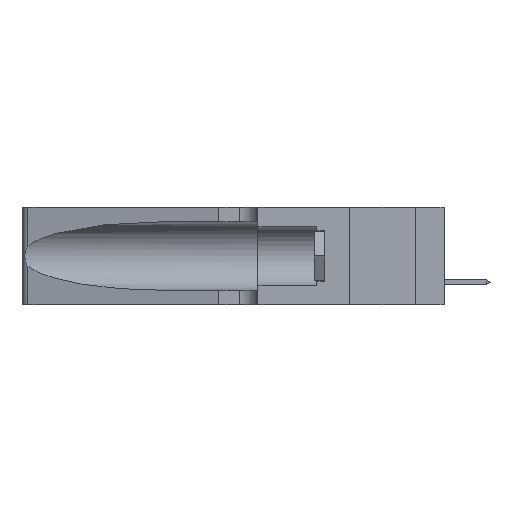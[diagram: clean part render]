
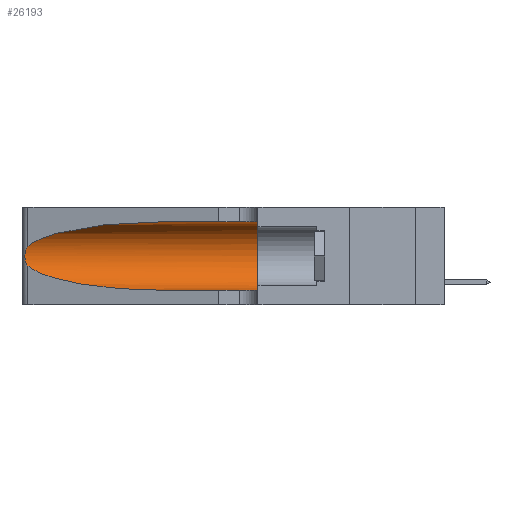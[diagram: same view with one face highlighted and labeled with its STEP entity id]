
A CAD part, left-side view. The second image highlights one B-rep face of the part: STEP entity #26193.
In plain terms, the highlighted cylindrical face has radius 3.308 mm (diameter 6.617 mm), a partial arc.
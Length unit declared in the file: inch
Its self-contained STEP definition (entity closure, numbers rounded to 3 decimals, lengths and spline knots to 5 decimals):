
#1196 = DIRECTION ( 'NONE',  ( 0., 0., -1. ) ) ;
#1380 = VERTEX_POINT ( 'NONE', #15927 ) ;
#1397 = CARTESIAN_POINT ( 'NONE',  ( 0.1305, 1.61858, 0.185 ) ) ;
#1692 = CARTESIAN_POINT ( 'NONE',  ( 0.26075, 1.23896, 0.19203 ) ) ;
#4645 = DIRECTION ( 'NONE',  ( 0., 0., 1. ) ) ;
#4853 = CYLINDRICAL_SURFACE ( 'NONE', #7527, 0.13025 ) ;
#5171 = CIRCLE ( 'NONE', #34325, 0.13025 ) ;
#5528 = DIRECTION ( 'NONE',  ( 0., -1., 0. ) ) ;
#6163 = FACE_OUTER_BOUND ( 'NONE', #28366, .T. ) ;
#6665 = CARTESIAN_POINT ( 'NONE',  ( 0.25487, 1.22718, 0.14631 ) ) ;
#7006 = ORIENTED_EDGE ( 'NONE', *, *, #47907, .F. ) ;
#7014 = CARTESIAN_POINT ( 'NONE',  ( 0.1305, 0.72297, 0.05475 ) ) ;
#7527 = AXIS2_PLACEMENT_3D ( 'NONE', #1397, #5528, #1196 ) ;
#8422 = VECTOR ( 'NONE', #16649, 39.37008 ) ;
#8935 = ORIENTED_EDGE ( 'NONE', *, *, #40357, .T. ) ;
#9298 = CARTESIAN_POINT ( 'NONE',  ( 0.25854, 1.2359, 0.20912 ) ) ;
#9604 = LINE ( 'NONE', #40719, #8422 ) ;
#10408 = CARTESIAN_POINT ( 'NONE',  ( 0.25639, 1.23186, 0.15144 ) ) ;
#10479 = CARTESIAN_POINT ( 'NONE',  ( 0.2373, 1.15595, 0.08982 ) ) ;
#14784 = VECTOR ( 'NONE', #36353, 39.37008 ) ;
#14871 = ORIENTED_EDGE ( 'NONE', *, *, #18354, .T. ) ;
#15927 = CARTESIAN_POINT ( 'NONE',  ( 0.1305, 0.35, 0.31525 ) ) ;
#16649 = DIRECTION ( 'NONE',  ( 0., -1., 0. ) ) ;
#17592 = ORIENTED_EDGE ( 'NONE', *, *, #23534, .F. ) ;
#18354 = EDGE_CURVE ( 'NONE', #25100, #36567, #29263, .T. ) ;
#18367 = CARTESIAN_POINT ( 'NONE',  ( 0.1305, 0.35, 0.05475 ) ) ;
#18776 = VERTEX_POINT ( 'NONE', #18367 ) ;
#19027 = CARTESIAN_POINT ( 'NONE',  ( 0.1305, 0.35, 0.185 ) ) ;
#19203 = CARTESIAN_POINT ( 'NONE',  ( 0.1305, 0.72297, 0.31525 ) ) ;
#20966 = CARTESIAN_POINT ( 'NONE',  ( 0.25555, 1.22994, 0.2215 ) ) ;
#21393 = VERTEX_POINT ( 'NONE', #7014 ) ;
#22049 = CARTESIAN_POINT ( 'NONE',  ( 0.25487, 1.22718, 0.14631 ) ) ;
#22215 = CARTESIAN_POINT ( 'NONE',  ( 0.26017, 1.23833, 0.17102 ) ) ;
#23534 = EDGE_CURVE ( 'NONE', #1380, #18776, #5171, .T. ) ;
#23563 = ORIENTED_EDGE ( 'NONE', *, *, #32424, .T. ) ;
#24275 = CARTESIAN_POINT ( 'NONE',  ( 0.1305, 0.72297, 0.31525 ) ) ;
#24586 = CARTESIAN_POINT ( 'NONE',  ( 0.25787, 1.23484, 0.2124 ) ) ;
#25100 = VERTEX_POINT ( 'NONE', #19203 ) ;
#25912 = CARTESIAN_POINT ( 'NONE',  ( 0.26018, 1.23835, 0.19895 ) ) ;
#26193 = ADVANCED_FACE ( 'NONE', ( #6163 ), #4853, .F. ) ;
#26478 = CARTESIAN_POINT ( 'NONE',  ( 0.26075, 1.23896, 0.178 ) ) ;
#26738 = CARTESIAN_POINT ( 'NONE',  ( 0.18966, 0.96281, 0.05475 ) ) ;
#26743 = CARTESIAN_POINT ( 'NONE',  ( 0.25487, 1.22718, 0.14631 ) ) ;
#28366 = EDGE_LOOP ( 'NONE', ( #14871, #28867, #23563, #8935, #17592, #7006 ) ) ;
#28867 = ORIENTED_EDGE ( 'NONE', *, *, #41584, .T. ) ;
#29263 =( BOUNDED_CURVE ( )  B_SPLINE_CURVE ( 3, ( #24275, #47881, #44480, #51704 ),
 .UNSPECIFIED., .F., .F. ) 
 B_SPLINE_CURVE_WITH_KNOTS ( ( 4, 4 ),
 ( 1.5708, 2.84003 ),
 .UNSPECIFIED. ) 
 CURVE ( )  GEOMETRIC_REPRESENTATION_ITEM ( )  RATIONAL_B_SPLINE_CURVE ( ( 1., 0.87, 0.87, 1. ) ) 
 REPRESENTATION_ITEM ( '' )  );
#30512 = CARTESIAN_POINT ( 'NONE',  ( 0.25856, 1.23593, 0.16098 ) ) ;
#30719 = CARTESIAN_POINT ( 'NONE',  ( 0.25789, 1.23486, 0.15765 ) ) ;
#30879 = CARTESIAN_POINT ( 'NONE',  ( 0.25487, 1.22718, 0.22369 ) ) ;
#32424 = EDGE_CURVE ( 'NONE', #36485, #21393, #37914, .T. ) ;
#34090 = B_SPLINE_CURVE_WITH_KNOTS ( 'NONE', 3,
 ( #37281, #20966, #37107, #24586, #9298, #25912, #1692, #26478, #22215, #30512, #30719, #10408, #35967, #26743 ),
 .UNSPECIFIED., .F., .F.,
 ( 4, 2, 2, 2, 2, 2, 4 ),
 ( 0., 0.00027, 0.00053, 0.00107, 0.0016, 0.00187, 0.00214 ),
 .UNSPECIFIED. ) ;
#34325 = AXIS2_PLACEMENT_3D ( 'NONE', #19027, #44220, #4645 ) ;
#34951 = CARTESIAN_POINT ( 'NONE',  ( 0.1305, 0.72297, 0.05475 ) ) ;
#35967 = CARTESIAN_POINT ( 'NONE',  ( 0.25555, 1.22993, 0.14849 ) ) ;
#36195 = LINE ( 'NONE', #44667, #14784 ) ;
#36353 = DIRECTION ( 'NONE',  ( 0., -1., 0. ) ) ;
#36485 = VERTEX_POINT ( 'NONE', #22049 ) ;
#36567 = VERTEX_POINT ( 'NONE', #30879 ) ;
#37107 = CARTESIAN_POINT ( 'NONE',  ( 0.25639, 1.23184, 0.21858 ) ) ;
#37281 = CARTESIAN_POINT ( 'NONE',  ( 0.25487, 1.22718, 0.22369 ) ) ;
#37914 =( BOUNDED_CURVE ( )  B_SPLINE_CURVE ( 3, ( #6665, #10479, #26738, #34951 ),
 .UNSPECIFIED., .F., .T. ) 
 B_SPLINE_CURVE_WITH_KNOTS ( ( 4, 4 ),
 ( 3.44316, 4.71239 ),
 .UNSPECIFIED. ) 
 CURVE ( )  GEOMETRIC_REPRESENTATION_ITEM ( )  RATIONAL_B_SPLINE_CURVE ( ( 1., 0.87, 0.87, 1. ) ) 
 REPRESENTATION_ITEM ( '' )  );
#40357 = EDGE_CURVE ( 'NONE', #21393, #18776, #36195, .T. ) ;
#40719 = CARTESIAN_POINT ( 'NONE',  ( 0.1305, 1.61858, 0.31525 ) ) ;
#41584 = EDGE_CURVE ( 'NONE', #36567, #36485, #34090, .T. ) ;
#44220 = DIRECTION ( 'NONE',  ( 0., 1., 0. ) ) ;
#44480 = CARTESIAN_POINT ( 'NONE',  ( 0.2373, 1.15595, 0.28018 ) ) ;
#44667 = CARTESIAN_POINT ( 'NONE',  ( 0.1305, 1.61858, 0.05475 ) ) ;
#47881 = CARTESIAN_POINT ( 'NONE',  ( 0.18966, 0.96281, 0.31525 ) ) ;
#47907 = EDGE_CURVE ( 'NONE', #25100, #1380, #9604, .T. ) ;
#51704 = CARTESIAN_POINT ( 'NONE',  ( 0.25487, 1.22718, 0.22369 ) ) ;
